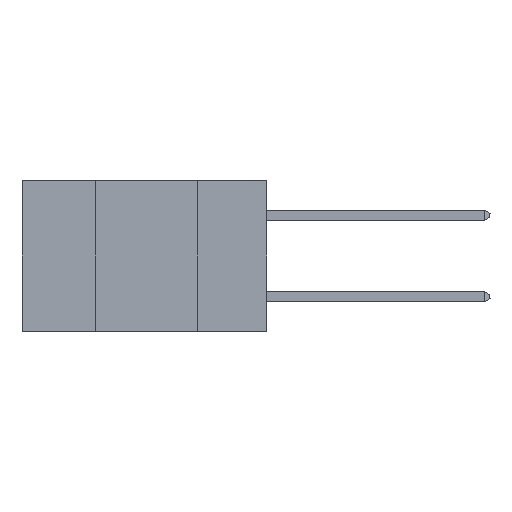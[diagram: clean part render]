
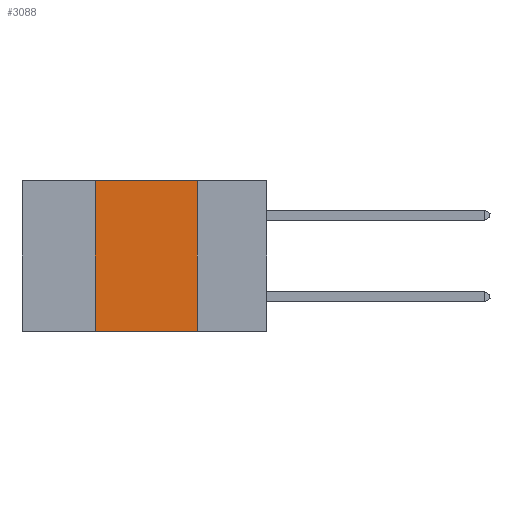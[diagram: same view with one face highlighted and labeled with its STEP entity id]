
A CAD part, left-side view. The second image highlights one B-rep face of the part: STEP entity #3088.
In plain terms, the highlighted planar face has unit normal (-1, 0, 0).
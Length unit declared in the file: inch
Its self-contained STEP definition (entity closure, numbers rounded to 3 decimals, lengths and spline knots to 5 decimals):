
#1233 = PLANE ( 'NONE',  #27811 ) ;
#3088 = ADVANCED_FACE ( 'NONE', ( #25039 ), #1233, .F. ) ;
#3914 = CARTESIAN_POINT ( 'NONE',  ( 0., 0.6, 0. ) ) ;
#4209 = VECTOR ( 'NONE', #9666, 39.37008 ) ;
#4496 = DIRECTION ( 'NONE',  ( 0., 0., -1. ) ) ;
#4981 = ORIENTED_EDGE ( 'NONE', *, *, #23369, .F. ) ;
#6281 = DIRECTION ( 'NONE',  ( 0., -1., 0. ) ) ;
#6316 = ORIENTED_EDGE ( 'NONE', *, *, #25230, .F. ) ;
#6467 = VECTOR ( 'NONE', #6281, 39.37008 ) ;
#6542 = VERTEX_POINT ( 'NONE', #23596 ) ;
#7003 = CARTESIAN_POINT ( 'NONE',  ( 0., 0.6, -0.37 ) ) ;
#9411 = CARTESIAN_POINT ( 'NONE',  ( 0., 0.42, -0.37 ) ) ;
#9666 = DIRECTION ( 'NONE',  ( 0., -1., 0. ) ) ;
#12236 = CARTESIAN_POINT ( 'NONE',  ( 0., 0.42, 0. ) ) ;
#13186 = DIRECTION ( 'NONE',  ( 0., 0., 1. ) ) ;
#13371 = EDGE_CURVE ( 'NONE', #20885, #20146, #24151, .T. ) ;
#13616 = EDGE_CURVE ( 'NONE', #20885, #6542, #18318, .T. ) ;
#14193 = CARTESIAN_POINT ( 'NONE',  ( 0., 0.17, 0. ) ) ;
#18318 = LINE ( 'NONE', #7003, #4209 ) ;
#19070 = DIRECTION ( 'NONE',  ( 0., 0., -1. ) ) ;
#19626 = CARTESIAN_POINT ( 'NONE',  ( 0., 0.6, 0. ) ) ;
#20146 = VERTEX_POINT ( 'NONE', #32091 ) ;
#20470 = EDGE_LOOP ( 'NONE', ( #4981, #6316, #25699, #25201 ) ) ;
#20885 = VERTEX_POINT ( 'NONE', #9411 ) ;
#21858 = CARTESIAN_POINT ( 'NONE',  ( 0., 0.17, 0. ) ) ;
#22462 = DIRECTION ( 'NONE',  ( 1., 0., 0. ) ) ;
#23343 = VECTOR ( 'NONE', #13186, 39.37008 ) ;
#23369 = EDGE_CURVE ( 'NONE', #27990, #6542, #30278, .T. ) ;
#23596 = CARTESIAN_POINT ( 'NONE',  ( 0., 0.17, -0.37 ) ) ;
#24151 = LINE ( 'NONE', #12236, #23343 ) ;
#25039 = FACE_OUTER_BOUND ( 'NONE', #20470, .T. ) ;
#25201 = ORIENTED_EDGE ( 'NONE', *, *, #13616, .T. ) ;
#25230 = EDGE_CURVE ( 'NONE', #20146, #27990, #28914, .T. ) ;
#25699 = ORIENTED_EDGE ( 'NONE', *, *, #13371, .F. ) ;
#27811 = AXIS2_PLACEMENT_3D ( 'NONE', #3914, #22462, #4496 ) ;
#27990 = VERTEX_POINT ( 'NONE', #21858 ) ;
#28914 = LINE ( 'NONE', #19626, #6467 ) ;
#30278 = LINE ( 'NONE', #14193, #31957 ) ;
#31957 = VECTOR ( 'NONE', #19070, 39.37008 ) ;
#32091 = CARTESIAN_POINT ( 'NONE',  ( 0., 0.42, 0. ) ) ;
